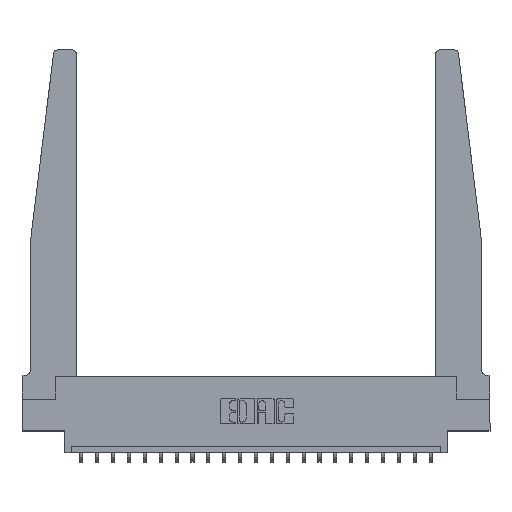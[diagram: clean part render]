
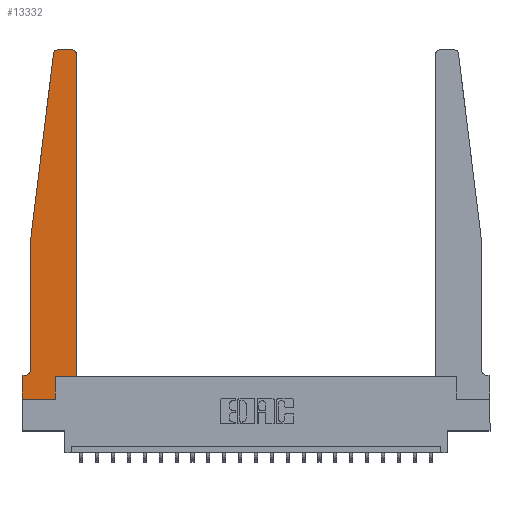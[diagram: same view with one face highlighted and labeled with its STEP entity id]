
A CAD part, top view. The second image highlights one B-rep face of the part: STEP entity #13332.
In plain terms, the highlighted planar face has unit normal (0, 0, 1).
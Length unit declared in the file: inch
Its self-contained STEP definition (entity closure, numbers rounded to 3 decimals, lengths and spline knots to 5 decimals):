
#85 = DIRECTION ( 'NONE',  ( 0., 0., 1. ) ) ;
#201 = DIRECTION ( 'NONE',  ( 1., 0., 0. ) ) ;
#268 = VERTEX_POINT ( 'NONE', #19919 ) ;
#337 = VECTOR ( 'NONE', #6212, 39.37008 ) ;
#520 = LINE ( 'NONE', #14218, #1781 ) ;
#529 = CARTESIAN_POINT ( 'NONE',  ( 0., 0., 0.37 ) ) ;
#787 = VERTEX_POINT ( 'NONE', #11216 ) ;
#1388 = EDGE_CURVE ( 'NONE', #787, #17300, #10241, .T. ) ;
#1548 = CARTESIAN_POINT ( 'NONE',  ( 0., 0., 0.37 ) ) ;
#1722 = AXIS2_PLACEMENT_3D ( 'NONE', #9229, #17680, #8909 ) ;
#1781 = VECTOR ( 'NONE', #7586, 39.37008 ) ;
#1842 = ORIENTED_EDGE ( 'NONE', *, *, #5003, .T. ) ;
#1883 = FACE_OUTER_BOUND ( 'NONE', #11953, .T. ) ;
#1967 = CARTESIAN_POINT ( 'NONE',  ( 0.25, 2.75, 0.37 ) ) ;
#2008 = ORIENTED_EDGE ( 'NONE', *, *, #6927, .T. ) ;
#2178 = AXIS2_PLACEMENT_3D ( 'NONE', #19923, #18222, #2466 ) ;
#2188 = DIRECTION ( 'NONE',  ( -1., 0., 0. ) ) ;
#2350 = CARTESIAN_POINT ( 'NONE',  ( 0.2605, 0.18, 0.37 ) ) ;
#2466 = DIRECTION ( 'NONE',  ( 1., 0., 0. ) ) ;
#2475 = VERTEX_POINT ( 'NONE', #5131 ) ;
#2847 = VECTOR ( 'NONE', #18935, 39.37008 ) ;
#2966 = CARTESIAN_POINT ( 'NONE',  ( 0.425, 0.18, 0.37 ) ) ;
#3016 = VECTOR ( 'NONE', #18160, 39.37008 ) ;
#3090 = EDGE_CURVE ( 'NONE', #14887, #787, #18375, .T. ) ;
#3240 = DIRECTION ( 'NONE',  ( 0., -1., 0. ) ) ;
#3433 = VERTEX_POINT ( 'NONE', #13451 ) ;
#3965 = ORIENTED_EDGE ( 'NONE', *, *, #9451, .T. ) ;
#4412 = VECTOR ( 'NONE', #2188, 39.37008 ) ;
#4514 = ORIENTED_EDGE ( 'NONE', *, *, #12039, .T. ) ;
#4629 = VERTEX_POINT ( 'NONE', #17717 ) ;
#5003 = EDGE_CURVE ( 'NONE', #10236, #4629, #19576, .T. ) ;
#5131 = CARTESIAN_POINT ( 'NONE',  ( 0.395, 2.75, 0.37 ) ) ;
#5358 = CARTESIAN_POINT ( 'NONE',  ( 0., 0.1875, 0.37 ) ) ;
#5894 = AXIS2_PLACEMENT_3D ( 'NONE', #17418, #16676, #6957 ) ;
#5935 = EDGE_CURVE ( 'NONE', #12502, #14887, #520, .T. ) ;
#6013 = DIRECTION ( 'NONE',  ( 1., 0., 0. ) ) ;
#6136 = ORIENTED_EDGE ( 'NONE', *, *, #12866, .T. ) ;
#6212 = DIRECTION ( 'NONE',  ( 1., 0., 0. ) ) ;
#6927 = EDGE_CURVE ( 'NONE', #17300, #2475, #10063, .T. ) ;
#6957 = DIRECTION ( 'NONE',  ( -1., 0., 0. ) ) ;
#7297 = VECTOR ( 'NONE', #22039, 39.37008 ) ;
#7394 = DIRECTION ( 'NONE',  ( -1., 0., 0. ) ) ;
#7586 = DIRECTION ( 'NONE',  ( 0., 1., 0. ) ) ;
#7834 = CIRCLE ( 'NONE', #1722, 0.03 ) ;
#8207 = VECTOR ( 'NONE', #7394, 39.37008 ) ;
#8421 = AXIS2_PLACEMENT_3D ( 'NONE', #5358, #85, #201 ) ;
#8730 = CARTESIAN_POINT ( 'NONE',  ( 0.065, 1.25, 0.37 ) ) ;
#8808 = CARTESIAN_POINT ( 'NONE',  ( 0.065, 1.25, 0.37 ) ) ;
#8909 = DIRECTION ( 'NONE',  ( 1., 0., 0. ) ) ;
#9211 = ORIENTED_EDGE ( 'NONE', *, *, #17631, .T. ) ;
#9229 = CARTESIAN_POINT ( 'NONE',  ( 0.27653, 2.72, 0.37 ) ) ;
#9451 = EDGE_CURVE ( 'NONE', #2475, #3433, #12079, .T. ) ;
#9861 = CIRCLE ( 'NONE', #5894, 0.05 ) ;
#10063 = CIRCLE ( 'NONE', #2178, 0.03 ) ;
#10091 = LINE ( 'NONE', #1548, #14970 ) ;
#10149 = VERTEX_POINT ( 'NONE', #11807 ) ;
#10225 = CARTESIAN_POINT ( 'NONE',  ( 0.24675, 2.72367, 0.37 ) ) ;
#10236 = VERTEX_POINT ( 'NONE', #10225 ) ;
#10241 = LINE ( 'NONE', #14777, #3016 ) ;
#10700 = ORIENTED_EDGE ( 'NONE', *, *, #1388, .T. ) ;
#11216 = CARTESIAN_POINT ( 'NONE',  ( 0.425, 0.18, 0.37 ) ) ;
#11807 = CARTESIAN_POINT ( 'NONE',  ( 0.015, 0.1875, 0.37 ) ) ;
#11953 = EDGE_LOOP ( 'NONE', ( #3965, #21002, #1842, #4514, #6136, #19890, #9211, #19521, #19621, #12449, #10700, #2008 ) ) ;
#12039 = EDGE_CURVE ( 'NONE', #4629, #13741, #15260, .T. ) ;
#12079 = LINE ( 'NONE', #1967, #4412 ) ;
#12449 = ORIENTED_EDGE ( 'NONE', *, *, #3090, .T. ) ;
#12502 = VERTEX_POINT ( 'NONE', #13418 ) ;
#12866 = EDGE_CURVE ( 'NONE', #13741, #10149, #9861, .T. ) ;
#13332 = ADVANCED_FACE ( 'NONE', ( #1883 ), #20455, .T. ) ;
#13418 = CARTESIAN_POINT ( 'NONE',  ( 0.2605, 0., 0.37 ) ) ;
#13451 = CARTESIAN_POINT ( 'NONE',  ( 0.27653, 2.75, 0.37 ) ) ;
#13581 = CARTESIAN_POINT ( 'NONE',  ( 0.425, 2.72, 0.37 ) ) ;
#13741 = VERTEX_POINT ( 'NONE', #17141 ) ;
#14218 = CARTESIAN_POINT ( 'NONE',  ( 0.2605, 0.18, 0.37 ) ) ;
#14777 = CARTESIAN_POINT ( 'NONE',  ( 0.425, 0.18, 0.37 ) ) ;
#14887 = VERTEX_POINT ( 'NONE', #2350 ) ;
#14970 = VECTOR ( 'NONE', #3240, 39.37008 ) ;
#15260 = LINE ( 'NONE', #8730, #7297 ) ;
#15729 = CARTESIAN_POINT ( 'NONE',  ( 0.065, 0.1875, 0.37 ) ) ;
#15955 = LINE ( 'NONE', #15729, #8207 ) ;
#16039 = LINE ( 'NONE', #529, #18671 ) ;
#16301 = EDGE_CURVE ( 'NONE', #10149, #268, #15955, .T. ) ;
#16490 = VERTEX_POINT ( 'NONE', #17055 ) ;
#16676 = DIRECTION ( 'NONE',  ( 0., 0., -1. ) ) ;
#17055 = CARTESIAN_POINT ( 'NONE',  ( 0., 0., 0.37 ) ) ;
#17141 = CARTESIAN_POINT ( 'NONE',  ( 0.065, 0.2375, 0.37 ) ) ;
#17300 = VERTEX_POINT ( 'NONE', #13581 ) ;
#17418 = CARTESIAN_POINT ( 'NONE',  ( 0.015, 0.2375, 0.37 ) ) ;
#17631 = EDGE_CURVE ( 'NONE', #268, #16490, #10091, .T. ) ;
#17680 = DIRECTION ( 'NONE',  ( 0., 0., 1. ) ) ;
#17717 = CARTESIAN_POINT ( 'NONE',  ( 0.065, 1.25, 0.37 ) ) ;
#18160 = DIRECTION ( 'NONE',  ( 0., 1., 0. ) ) ;
#18222 = DIRECTION ( 'NONE',  ( 0., 0., 1. ) ) ;
#18375 = LINE ( 'NONE', #2966, #337 ) ;
#18671 = VECTOR ( 'NONE', #6013, 39.37008 ) ;
#18720 = EDGE_CURVE ( 'NONE', #3433, #10236, #7834, .T. ) ;
#18935 = DIRECTION ( 'NONE',  ( -0.122, -0.992, 0. ) ) ;
#19521 = ORIENTED_EDGE ( 'NONE', *, *, #20636, .T. ) ;
#19576 = LINE ( 'NONE', #8808, #2847 ) ;
#19621 = ORIENTED_EDGE ( 'NONE', *, *, #5935, .T. ) ;
#19890 = ORIENTED_EDGE ( 'NONE', *, *, #16301, .T. ) ;
#19919 = CARTESIAN_POINT ( 'NONE',  ( 0., 0.1875, 0.37 ) ) ;
#19923 = CARTESIAN_POINT ( 'NONE',  ( 0.395, 2.72, 0.37 ) ) ;
#20455 = PLANE ( 'NONE',  #8421 ) ;
#20636 = EDGE_CURVE ( 'NONE', #16490, #12502, #16039, .T. ) ;
#21002 = ORIENTED_EDGE ( 'NONE', *, *, #18720, .T. ) ;
#22039 = DIRECTION ( 'NONE',  ( 0., -1., 0. ) ) ;
